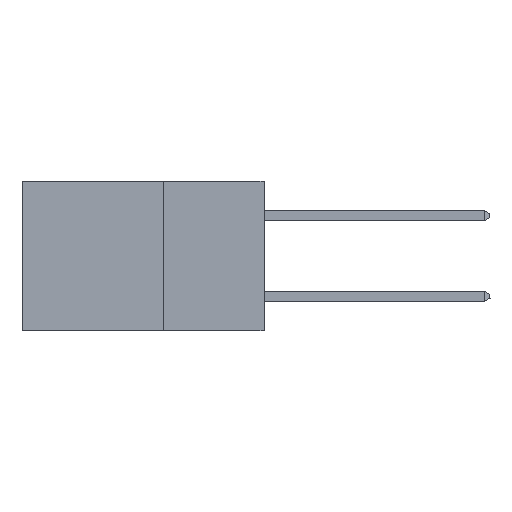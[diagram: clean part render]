
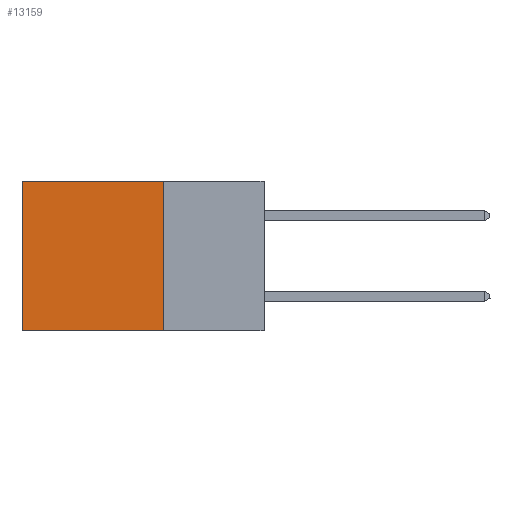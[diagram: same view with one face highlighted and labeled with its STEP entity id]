
A CAD part, left-side view. The second image highlights one B-rep face of the part: STEP entity #13159.
In plain terms, the highlighted planar face has unit normal (-1, 0, 0).
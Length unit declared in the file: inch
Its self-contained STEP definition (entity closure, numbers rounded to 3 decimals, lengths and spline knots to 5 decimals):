
#1900 = DIRECTION ( 'NONE',  ( 0., 0., -1. ) ) ;
#2438 = AXIS2_PLACEMENT_3D ( 'NONE', #9896, #18547, #5548 ) ;
#2862 = DIRECTION ( 'NONE',  ( 0., 1., 0. ) ) ;
#3287 = PLANE ( 'NONE',  #2438 ) ;
#4866 = EDGE_CURVE ( 'NONE', #24114, #15719, #6428, .T. ) ;
#4890 = ORIENTED_EDGE ( 'NONE', *, *, #17030, .T. ) ;
#5028 = VECTOR ( 'NONE', #2862, 39.37008 ) ;
#5548 = DIRECTION ( 'NONE',  ( 0., 0., -1. ) ) ;
#6428 = LINE ( 'NONE', #12919, #5028 ) ;
#8096 = EDGE_CURVE ( 'NONE', #14963, #24114, #27090, .T. ) ;
#8614 = CARTESIAN_POINT ( 'NONE',  ( 0.298, 0.25, 0. ) ) ;
#9896 = CARTESIAN_POINT ( 'NONE',  ( 0.298, 0.25, 0. ) ) ;
#10990 = CARTESIAN_POINT ( 'NONE',  ( 0.298, 0.6, 0. ) ) ;
#11637 = ORIENTED_EDGE ( 'NONE', *, *, #20368, .T. ) ;
#12296 = CARTESIAN_POINT ( 'NONE',  ( 0.298, 0.25, 0. ) ) ;
#12919 = CARTESIAN_POINT ( 'NONE',  ( 0.298, 0.25, -0.37 ) ) ;
#13159 = ADVANCED_FACE ( 'NONE', ( #19629 ), #3287, .F. ) ;
#13318 = CARTESIAN_POINT ( 'NONE',  ( 0.298, 0.25, -0.37 ) ) ;
#14649 = VECTOR ( 'NONE', #27919, 39.37008 ) ;
#14963 = VERTEX_POINT ( 'NONE', #12296 ) ;
#15719 = VERTEX_POINT ( 'NONE', #17214 ) ;
#15896 = EDGE_LOOP ( 'NONE', ( #11637, #21802, #27777, #4890 ) ) ;
#16125 = VECTOR ( 'NONE', #27819, 39.37008 ) ;
#16762 = CARTESIAN_POINT ( 'NONE',  ( 0.298, 0.6, 0. ) ) ;
#17030 = EDGE_CURVE ( 'NONE', #14963, #22715, #18861, .T. ) ;
#17168 = CARTESIAN_POINT ( 'NONE',  ( 0.298, 0.25, 0. ) ) ;
#17214 = CARTESIAN_POINT ( 'NONE',  ( 0.298, 0.6, -0.37 ) ) ;
#18547 = DIRECTION ( 'NONE',  ( 1., 0., 0. ) ) ;
#18861 = LINE ( 'NONE', #17168, #16125 ) ;
#19629 = FACE_OUTER_BOUND ( 'NONE', #15896, .T. ) ;
#20368 = EDGE_CURVE ( 'NONE', #22715, #15719, #21047, .T. ) ;
#21047 = LINE ( 'NONE', #10990, #14649 ) ;
#21802 = ORIENTED_EDGE ( 'NONE', *, *, #4866, .F. ) ;
#22715 = VERTEX_POINT ( 'NONE', #16762 ) ;
#24114 = VERTEX_POINT ( 'NONE', #13318 ) ;
#26416 = VECTOR ( 'NONE', #1900, 39.37008 ) ;
#27090 = LINE ( 'NONE', #8614, #26416 ) ;
#27777 = ORIENTED_EDGE ( 'NONE', *, *, #8096, .F. ) ;
#27819 = DIRECTION ( 'NONE',  ( 0., 1., 0. ) ) ;
#27919 = DIRECTION ( 'NONE',  ( 0., 0., -1. ) ) ;
